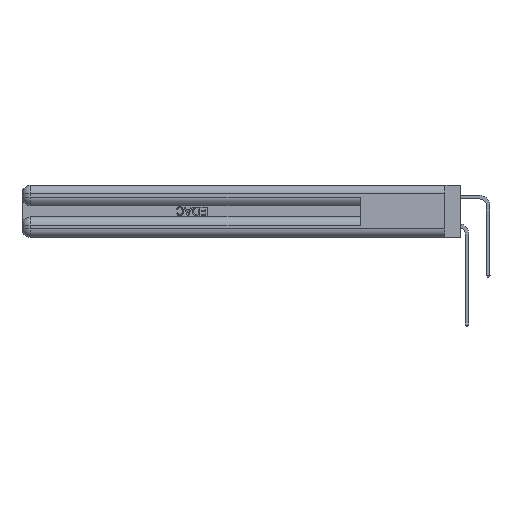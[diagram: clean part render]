
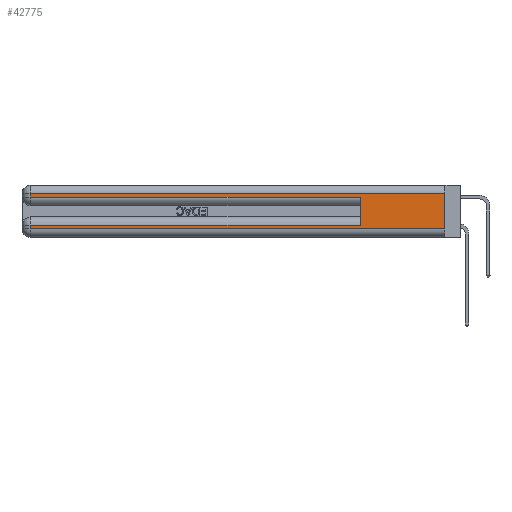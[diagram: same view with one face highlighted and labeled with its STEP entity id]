
A CAD part, left-side view. The second image highlights one B-rep face of the part: STEP entity #42775.
In plain terms, the highlighted planar face has unit normal (-1, 0, 0).
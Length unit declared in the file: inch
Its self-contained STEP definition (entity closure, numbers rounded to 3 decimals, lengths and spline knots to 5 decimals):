
#926 = CARTESIAN_POINT ( 'NONE',  ( 0., 2.94, 0.37 ) ) ;
#1188 = VECTOR ( 'NONE', #24106, 39.37008 ) ;
#1228 = CARTESIAN_POINT ( 'NONE',  ( 0., 2.94, 0.06 ) ) ;
#3234 = VECTOR ( 'NONE', #8335, 39.37008 ) ;
#3318 = LINE ( 'NONE', #8928, #30058 ) ;
#4518 = VECTOR ( 'NONE', #26736, 39.37008 ) ;
#4811 = CARTESIAN_POINT ( 'NONE',  ( 0., 0., 0.085 ) ) ;
#5428 = EDGE_CURVE ( 'NONE', #39897, #13254, #12968, .T. ) ;
#5885 = LINE ( 'NONE', #14317, #7044 ) ;
#6480 = ORIENTED_EDGE ( 'NONE', *, *, #37955, .T. ) ;
#7044 = VECTOR ( 'NONE', #39672, 39.37008 ) ;
#7126 = CARTESIAN_POINT ( 'NONE',  ( 0., 2.94, 0.31 ) ) ;
#7391 = DIRECTION ( 'NONE',  ( 0., 0., -1. ) ) ;
#8335 = DIRECTION ( 'NONE',  ( 0., 0., -1. ) ) ;
#8928 = CARTESIAN_POINT ( 'NONE',  ( 0., 0., 0.31 ) ) ;
#9475 = CARTESIAN_POINT ( 'NONE',  ( 0., 0., 0.37 ) ) ;
#10465 = ORIENTED_EDGE ( 'NONE', *, *, #5428, .T. ) ;
#10552 = VECTOR ( 'NONE', #27871, 39.37008 ) ;
#11874 = EDGE_CURVE ( 'NONE', #38356, #18470, #43167, .T. ) ;
#12102 = LINE ( 'NONE', #27728, #1188 ) ;
#12565 = DIRECTION ( 'NONE',  ( 0., 1., 0. ) ) ;
#12968 = LINE ( 'NONE', #22912, #3234 ) ;
#13097 = DIRECTION ( 'NONE',  ( 0., 0., -1. ) ) ;
#13254 = VERTEX_POINT ( 'NONE', #45708 ) ;
#14317 = CARTESIAN_POINT ( 'NONE',  ( 0., 0., 0.06 ) ) ;
#14801 = VERTEX_POINT ( 'NONE', #46366 ) ;
#15388 = CARTESIAN_POINT ( 'NONE',  ( 0., 0., 0.06 ) ) ;
#17622 = EDGE_CURVE ( 'NONE', #13254, #23115, #29825, .T. ) ;
#18228 = EDGE_CURVE ( 'NONE', #24976, #42392, #5885, .T. ) ;
#18470 = VERTEX_POINT ( 'NONE', #26985 ) ;
#22912 = CARTESIAN_POINT ( 'NONE',  ( 0., 2.94, 0.37 ) ) ;
#23055 = VECTOR ( 'NONE', #29919, 39.37008 ) ;
#23115 = VERTEX_POINT ( 'NONE', #37023 ) ;
#23391 = EDGE_CURVE ( 'NONE', #14801, #42392, #42646, .T. ) ;
#24106 = DIRECTION ( 'NONE',  ( 0., 0., 1. ) ) ;
#24109 = ORIENTED_EDGE ( 'NONE', *, *, #23391, .F. ) ;
#24258 = CARTESIAN_POINT ( 'NONE',  ( 0., 0., 0.285 ) ) ;
#24976 = VERTEX_POINT ( 'NONE', #1228 ) ;
#25332 = ORIENTED_EDGE ( 'NONE', *, *, #18228, .T. ) ;
#25510 = PLANE ( 'NONE',  #33955 ) ;
#26736 = DIRECTION ( 'NONE',  ( 0., 1., 0. ) ) ;
#26985 = CARTESIAN_POINT ( 'NONE',  ( 0., 2.94, 0.085 ) ) ;
#27728 = CARTESIAN_POINT ( 'NONE',  ( 0., 0.6, 0.145 ) ) ;
#27871 = DIRECTION ( 'NONE',  ( 0., -1., 0. ) ) ;
#28343 = CARTESIAN_POINT ( 'NONE',  ( 0., 0., 0.37 ) ) ;
#29147 = DIRECTION ( 'NONE',  ( 1., 0., 0. ) ) ;
#29263 = EDGE_LOOP ( 'NONE', ( #24109, #6480, #10465, #33142, #35396, #46285, #31560, #25332 ) ) ;
#29825 = LINE ( 'NONE', #24258, #10552 ) ;
#29919 = DIRECTION ( 'NONE',  ( 0., 0., -1. ) ) ;
#30058 = VECTOR ( 'NONE', #12565, 39.37008 ) ;
#30998 = FACE_OUTER_BOUND ( 'NONE', #29263, .T. ) ;
#31560 = ORIENTED_EDGE ( 'NONE', *, *, #33723, .T. ) ;
#31566 = LINE ( 'NONE', #926, #23055 ) ;
#33142 = ORIENTED_EDGE ( 'NONE', *, *, #17622, .T. ) ;
#33723 = EDGE_CURVE ( 'NONE', #18470, #24976, #31566, .T. ) ;
#33955 = AXIS2_PLACEMENT_3D ( 'NONE', #28343, #29147, #7391 ) ;
#34120 = VECTOR ( 'NONE', #13097, 39.37008 ) ;
#35396 = ORIENTED_EDGE ( 'NONE', *, *, #44350, .F. ) ;
#37023 = CARTESIAN_POINT ( 'NONE',  ( 0., 0.6, 0.285 ) ) ;
#37955 = EDGE_CURVE ( 'NONE', #14801, #39897, #3318, .T. ) ;
#38356 = VERTEX_POINT ( 'NONE', #43606 ) ;
#39672 = DIRECTION ( 'NONE',  ( 0., -1., 0. ) ) ;
#39897 = VERTEX_POINT ( 'NONE', #7126 ) ;
#42392 = VERTEX_POINT ( 'NONE', #15388 ) ;
#42646 = LINE ( 'NONE', #9475, #34120 ) ;
#42775 = ADVANCED_FACE ( 'NONE', ( #30998 ), #25510, .F. ) ;
#43167 = LINE ( 'NONE', #4811, #4518 ) ;
#43606 = CARTESIAN_POINT ( 'NONE',  ( 0., 0.6, 0.085 ) ) ;
#44350 = EDGE_CURVE ( 'NONE', #38356, #23115, #12102, .T. ) ;
#45708 = CARTESIAN_POINT ( 'NONE',  ( 0., 2.94, 0.285 ) ) ;
#46285 = ORIENTED_EDGE ( 'NONE', *, *, #11874, .T. ) ;
#46366 = CARTESIAN_POINT ( 'NONE',  ( 0., 0., 0.31 ) ) ;
